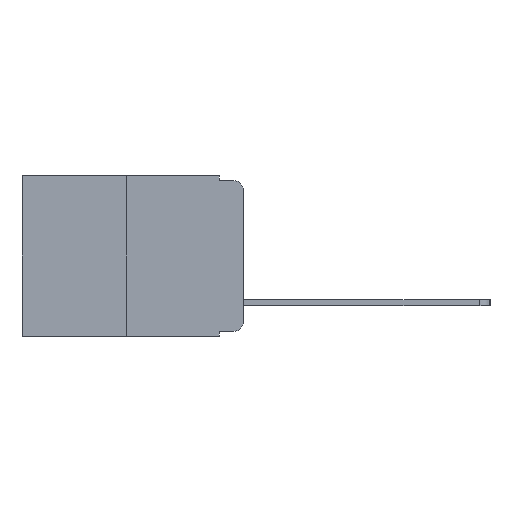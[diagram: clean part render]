
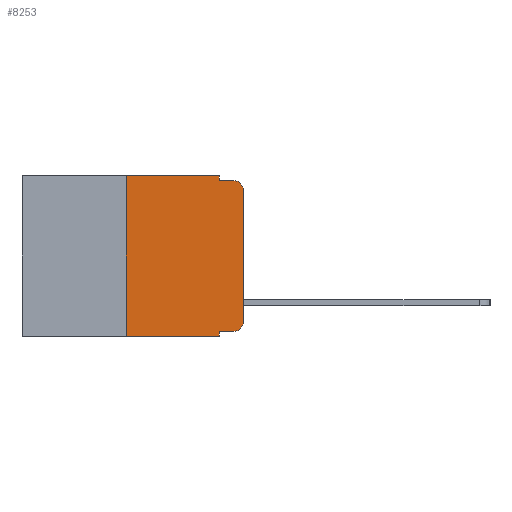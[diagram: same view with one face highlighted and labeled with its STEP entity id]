
A CAD part, left-side view. The second image highlights one B-rep face of the part: STEP entity #8253.
In plain terms, the highlighted planar face has unit normal (-1, 0, 0).
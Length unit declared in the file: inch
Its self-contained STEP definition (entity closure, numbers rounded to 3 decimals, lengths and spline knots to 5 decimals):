
#19 = VECTOR ( 'NONE', #19441, 39.37008 ) ;
#179 = CARTESIAN_POINT ( 'NONE',  ( 0., 0.473, -0.343 ) ) ;
#894 = ORIENTED_EDGE ( 'NONE', *, *, #14611, .F. ) ;
#1211 = CARTESIAN_POINT ( 'NONE',  ( 0., 0.25, 0. ) ) ;
#1350 = CARTESIAN_POINT ( 'NONE',  ( 0., 0.051, -0.01 ) ) ;
#1994 = ORIENTED_EDGE ( 'NONE', *, *, #16164, .T. ) ;
#2161 = VECTOR ( 'NONE', #3887, 39.37008 ) ;
#2231 = EDGE_LOOP ( 'NONE', ( #18556, #6381, #8047, #5081, #13879, #894, #9590, #16645, #6980, #1994 ) ) ;
#2270 = CARTESIAN_POINT ( 'NONE',  ( 0., 0.25, 0. ) ) ;
#2271 = VECTOR ( 'NONE', #9785, 39.37008 ) ;
#3368 = AXIS2_PLACEMENT_3D ( 'NONE', #18622, #20189, #10729 ) ;
#3422 = VERTEX_POINT ( 'NONE', #2270 ) ;
#3724 = LINE ( 'NONE', #5537, #2161 ) ;
#3786 = VECTOR ( 'NONE', #6477, 39.37008 ) ;
#3887 = DIRECTION ( 'NONE',  ( 0., -1., 0. ) ) ;
#4423 = LINE ( 'NONE', #9906, #19 ) ;
#4474 = VECTOR ( 'NONE', #20171, 39.37008 ) ;
#4553 = CARTESIAN_POINT ( 'NONE',  ( 0., 0.02, -0.01 ) ) ;
#5081 = ORIENTED_EDGE ( 'NONE', *, *, #16584, .F. ) ;
#5177 = DIRECTION ( 'NONE',  ( 0., -1., 0. ) ) ;
#5537 = CARTESIAN_POINT ( 'NONE',  ( 0., 0.051, -0.333 ) ) ;
#5702 = DIRECTION ( 'NONE',  ( -1., 0., 0. ) ) ;
#5987 = CARTESIAN_POINT ( 'NONE',  ( 0., 0.02, -0.333 ) ) ;
#6099 = VERTEX_POINT ( 'NONE', #5987 ) ;
#6127 = CARTESIAN_POINT ( 'NONE',  ( 0., 0., -0.03 ) ) ;
#6381 = ORIENTED_EDGE ( 'NONE', *, *, #14079, .T. ) ;
#6477 = DIRECTION ( 'NONE',  ( 0., -1., 0. ) ) ;
#6980 = ORIENTED_EDGE ( 'NONE', *, *, #8560, .T. ) ;
#7005 = CARTESIAN_POINT ( 'NONE',  ( 0., 0., -0.313 ) ) ;
#7103 = LINE ( 'NONE', #16167, #2271 ) ;
#7394 = CARTESIAN_POINT ( 'NONE',  ( 0., 0., 0. ) ) ;
#7918 = DIRECTION ( 'NONE',  ( 0., 0., 1. ) ) ;
#8047 = ORIENTED_EDGE ( 'NONE', *, *, #8713, .F. ) ;
#8119 = VERTEX_POINT ( 'NONE', #15114 ) ;
#8253 = ADVANCED_FACE ( 'NONE', ( #13524 ), #9098, .F. ) ;
#8560 = EDGE_CURVE ( 'NONE', #12556, #6099, #3724, .T. ) ;
#8713 = EDGE_CURVE ( 'NONE', #19547, #16348, #17718, .T. ) ;
#8721 = CIRCLE ( 'NONE', #9319, 0.02 ) ;
#8810 = DIRECTION ( 'NONE',  ( -1., 0., 0. ) ) ;
#9098 = PLANE ( 'NONE',  #3368 ) ;
#9319 = AXIS2_PLACEMENT_3D ( 'NONE', #15273, #5702, #16846 ) ;
#9590 = ORIENTED_EDGE ( 'NONE', *, *, #17264, .T. ) ;
#9785 = DIRECTION ( 'NONE',  ( 0., 0., -1. ) ) ;
#9906 = CARTESIAN_POINT ( 'NONE',  ( 0., 0.051, 0. ) ) ;
#10668 = CIRCLE ( 'NONE', #14660, 0.02 ) ;
#10729 = DIRECTION ( 'NONE',  ( 0., 0., -1. ) ) ;
#11415 = EDGE_CURVE ( 'NONE', #12556, #14682, #7103, .T. ) ;
#11959 = EDGE_CURVE ( 'NONE', #16695, #20070, #18172, .T. ) ;
#12401 = VECTOR ( 'NONE', #7918, 39.37008 ) ;
#12556 = VERTEX_POINT ( 'NONE', #20347 ) ;
#13524 = FACE_OUTER_BOUND ( 'NONE', #2231, .T. ) ;
#13605 = CARTESIAN_POINT ( 'NONE',  ( 0., 0.25, -0.343 ) ) ;
#13686 = VECTOR ( 'NONE', #5177, 39.37008 ) ;
#13879 = ORIENTED_EDGE ( 'NONE', *, *, #20247, .F. ) ;
#13982 = VECTOR ( 'NONE', #18527, 39.37008 ) ;
#14079 = EDGE_CURVE ( 'NONE', #20070, #16348, #10668, .T. ) ;
#14611 = EDGE_CURVE ( 'NONE', #15548, #3422, #20771, .T. ) ;
#14660 = AXIS2_PLACEMENT_3D ( 'NONE', #18319, #8810, #19894 ) ;
#14682 = VERTEX_POINT ( 'NONE', #19170 ) ;
#15114 = CARTESIAN_POINT ( 'NONE',  ( 0., 0.051, 0. ) ) ;
#15273 = CARTESIAN_POINT ( 'NONE',  ( 0., 0.02, -0.313 ) ) ;
#15548 = VERTEX_POINT ( 'NONE', #13605 ) ;
#16164 = EDGE_CURVE ( 'NONE', #6099, #16695, #8721, .T. ) ;
#16167 = CARTESIAN_POINT ( 'NONE',  ( 0., 0.051, 0. ) ) ;
#16348 = VERTEX_POINT ( 'NONE', #4553 ) ;
#16584 = EDGE_CURVE ( 'NONE', #8119, #19547, #4423, .T. ) ;
#16645 = ORIENTED_EDGE ( 'NONE', *, *, #11415, .F. ) ;
#16695 = VERTEX_POINT ( 'NONE', #7005 ) ;
#16846 = DIRECTION ( 'NONE',  ( 0., 0., -1. ) ) ;
#17264 = EDGE_CURVE ( 'NONE', #15548, #14682, #17888, .T. ) ;
#17620 = CARTESIAN_POINT ( 'NONE',  ( 0., 0.473, 0. ) ) ;
#17718 = LINE ( 'NONE', #18603, #4474 ) ;
#17888 = LINE ( 'NONE', #179, #13686 ) ;
#18172 = LINE ( 'NONE', #7394, #13982 ) ;
#18319 = CARTESIAN_POINT ( 'NONE',  ( 0., 0.02, -0.03 ) ) ;
#18527 = DIRECTION ( 'NONE',  ( 0., 0., 1. ) ) ;
#18556 = ORIENTED_EDGE ( 'NONE', *, *, #11959, .T. ) ;
#18603 = CARTESIAN_POINT ( 'NONE',  ( 0., 0.051, -0.01 ) ) ;
#18622 = CARTESIAN_POINT ( 'NONE',  ( 0., 0.473, 0. ) ) ;
#19170 = CARTESIAN_POINT ( 'NONE',  ( 0., 0.051, -0.343 ) ) ;
#19441 = DIRECTION ( 'NONE',  ( 0., 0., -1. ) ) ;
#19547 = VERTEX_POINT ( 'NONE', #1350 ) ;
#19894 = DIRECTION ( 'NONE',  ( 0., 0., -1. ) ) ;
#20070 = VERTEX_POINT ( 'NONE', #6127 ) ;
#20171 = DIRECTION ( 'NONE',  ( 0., -1., 0. ) ) ;
#20189 = DIRECTION ( 'NONE',  ( 1., 0., 0. ) ) ;
#20247 = EDGE_CURVE ( 'NONE', #3422, #8119, #20717, .T. ) ;
#20347 = CARTESIAN_POINT ( 'NONE',  ( 0., 0.051, -0.333 ) ) ;
#20717 = LINE ( 'NONE', #17620, #3786 ) ;
#20771 = LINE ( 'NONE', #1211, #12401 ) ;
